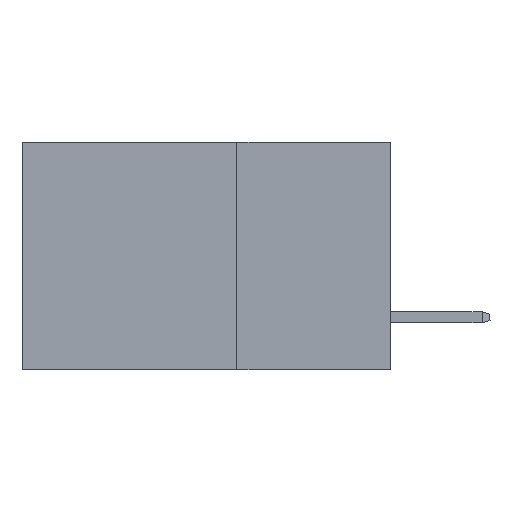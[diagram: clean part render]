
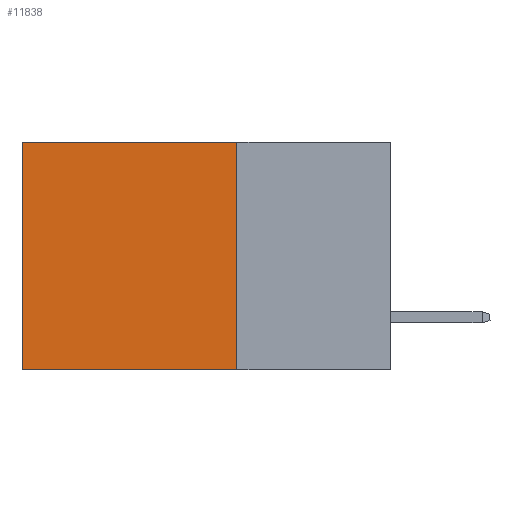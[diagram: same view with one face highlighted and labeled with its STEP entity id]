
A CAD part, left-side view. The second image highlights one B-rep face of the part: STEP entity #11838.
In plain terms, the highlighted planar face has unit normal (-1, 0, 0).
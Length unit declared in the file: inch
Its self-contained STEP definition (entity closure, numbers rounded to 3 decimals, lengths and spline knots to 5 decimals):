
#904 = AXIS2_PLACEMENT_3D ( 'NONE', #2292, #11483, #3697 ) ;
#1177 = EDGE_CURVE ( 'NONE', #9762, #16554, #6439, .T. ) ;
#1824 = VERTEX_POINT ( 'NONE', #3898 ) ;
#2292 = CARTESIAN_POINT ( 'NONE',  ( 0.2875, 0.25, 0. ) ) ;
#2297 = ORIENTED_EDGE ( 'NONE', *, *, #10667, .T. ) ;
#2720 = VECTOR ( 'NONE', #14035, 39.37008 ) ;
#2773 = VECTOR ( 'NONE', #11854, 39.37008 ) ;
#2886 = CARTESIAN_POINT ( 'NONE',  ( 0.2875, 0.6, -0.37 ) ) ;
#3199 = VECTOR ( 'NONE', #15613, 39.37008 ) ;
#3697 = DIRECTION ( 'NONE',  ( 0., 0., -1. ) ) ;
#3898 = CARTESIAN_POINT ( 'NONE',  ( 0.2875, 0.6, 0. ) ) ;
#4145 = CARTESIAN_POINT ( 'NONE',  ( 0.2875, 0.25, 0. ) ) ;
#6365 = LINE ( 'NONE', #11580, #2720 ) ;
#6408 = CARTESIAN_POINT ( 'NONE',  ( 0.2875, 0.25, 0. ) ) ;
#6439 = LINE ( 'NONE', #6408, #6894 ) ;
#6894 = VECTOR ( 'NONE', #8090, 39.37008 ) ;
#7240 = FACE_OUTER_BOUND ( 'NONE', #10750, .T. ) ;
#7244 = ORIENTED_EDGE ( 'NONE', *, *, #11911, .F. ) ;
#8090 = DIRECTION ( 'NONE',  ( 0., 0., -1. ) ) ;
#9019 = PLANE ( 'NONE',  #904 ) ;
#9538 = VERTEX_POINT ( 'NONE', #2886 ) ;
#9762 = VERTEX_POINT ( 'NONE', #14874 ) ;
#9898 = LINE ( 'NONE', #10680, #2773 ) ;
#10667 = EDGE_CURVE ( 'NONE', #1824, #9538, #9898, .T. ) ;
#10680 = CARTESIAN_POINT ( 'NONE',  ( 0.2875, 0.6, 0. ) ) ;
#10750 = EDGE_LOOP ( 'NONE', ( #2297, #7244, #14983, #12137 ) ) ;
#11053 = EDGE_CURVE ( 'NONE', #9762, #1824, #16735, .T. ) ;
#11483 = DIRECTION ( 'NONE',  ( 1., 0., 0. ) ) ;
#11580 = CARTESIAN_POINT ( 'NONE',  ( 0.2875, 0.25, -0.37 ) ) ;
#11838 = ADVANCED_FACE ( 'NONE', ( #7240 ), #9019, .F. ) ;
#11854 = DIRECTION ( 'NONE',  ( 0., 0., -1. ) ) ;
#11911 = EDGE_CURVE ( 'NONE', #16554, #9538, #6365, .T. ) ;
#12137 = ORIENTED_EDGE ( 'NONE', *, *, #11053, .T. ) ;
#12761 = CARTESIAN_POINT ( 'NONE',  ( 0.2875, 0.25, -0.37 ) ) ;
#14035 = DIRECTION ( 'NONE',  ( 0., 1., 0. ) ) ;
#14874 = CARTESIAN_POINT ( 'NONE',  ( 0.2875, 0.25, 0. ) ) ;
#14983 = ORIENTED_EDGE ( 'NONE', *, *, #1177, .F. ) ;
#15613 = DIRECTION ( 'NONE',  ( 0., 1., 0. ) ) ;
#16554 = VERTEX_POINT ( 'NONE', #12761 ) ;
#16735 = LINE ( 'NONE', #4145, #3199 ) ;
